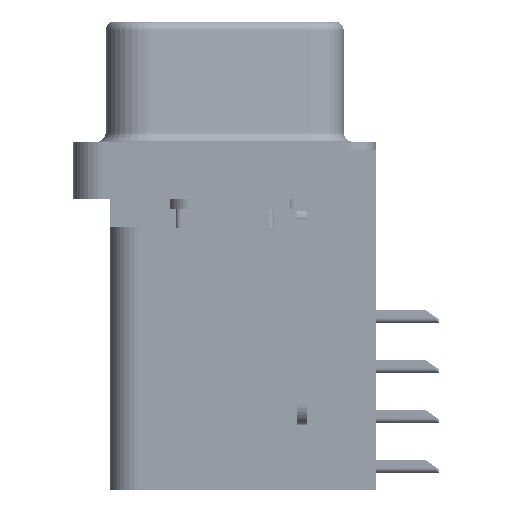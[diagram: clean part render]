
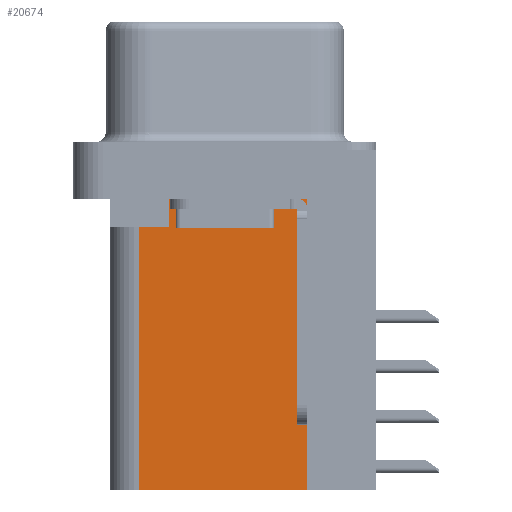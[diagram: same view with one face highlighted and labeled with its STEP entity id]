
A CAD part, left-side view. The second image highlights one B-rep face of the part: STEP entity #20674.
In plain terms, the highlighted planar face has unit normal (-1, 0, 0).
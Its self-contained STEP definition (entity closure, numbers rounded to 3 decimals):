
#11 = VECTOR ( 'NONE', #14169, 1000. ) ;
#483 = EDGE_CURVE ( 'NONE', #10959, #42456, #28727, .T. ) ;
#543 = LINE ( 'NONE', #10920, #11 ) ;
#1434 = DIRECTION ( 'NONE',  ( 0., 0., 1. ) ) ;
#1807 = CARTESIAN_POINT ( 'NONE',  ( 3.75, 2.85, -2.5 ) ) ;
#3070 = ORIENTED_EDGE ( 'NONE', *, *, #483, .F. ) ;
#3157 = CARTESIAN_POINT ( 'NONE',  ( 3.75, -4.2, -17.3 ) ) ;
#3309 = ORIENTED_EDGE ( 'NONE', *, *, #20589, .T. ) ;
#5395 = EDGE_CURVE ( 'NONE', #41770, #30241, #40877, .T. ) ;
#6801 = PLANE ( 'NONE',  #29331 ) ;
#7003 = EDGE_CURVE ( 'NONE', #41770, #10959, #31390, .T. ) ;
#8115 = CARTESIAN_POINT ( 'NONE',  ( 3.75, -4.2, -17.3 ) ) ;
#9763 = CARTESIAN_POINT ( 'NONE',  ( 3.75, -4.2, -2.5 ) ) ;
#10448 = DIRECTION ( 'NONE',  ( 0., 1., 0. ) ) ;
#10920 = CARTESIAN_POINT ( 'NONE',  ( 3.75, 2.85, -3.9 ) ) ;
#10959 = VERTEX_POINT ( 'NONE', #27523 ) ;
#12571 = CARTESIAN_POINT ( 'NONE',  ( 3.75, -4.2, -2.5 ) ) ;
#12845 = CARTESIAN_POINT ( 'NONE',  ( 3.75, 4.35, -17.3 ) ) ;
#13316 = CARTESIAN_POINT ( 'NONE',  ( 3.75, 2.85, -3.9 ) ) ;
#14169 = DIRECTION ( 'NONE',  ( 0., 0., -1. ) ) ;
#15286 = LINE ( 'NONE', #29751, #15405 ) ;
#15405 = VECTOR ( 'NONE', #10448, 1000. ) ;
#16669 = DIRECTION ( 'NONE',  ( 0., 1., 0. ) ) ;
#19621 = FACE_OUTER_BOUND ( 'NONE', #41971, .T. ) ;
#20589 = EDGE_CURVE ( 'NONE', #30241, #28716, #21363, .T. ) ;
#20674 = ADVANCED_FACE ( 'NONE', ( #19621 ), #6801, .F. ) ;
#21363 = LINE ( 'NONE', #9763, #21682 ) ;
#21682 = VECTOR ( 'NONE', #42004, 1000. ) ;
#22432 = ORIENTED_EDGE ( 'NONE', *, *, #24469, .T. ) ;
#22779 = VERTEX_POINT ( 'NONE', #13316 ) ;
#22908 = EDGE_CURVE ( 'NONE', #28716, #22779, #543, .T. ) ;
#23600 = ORIENTED_EDGE ( 'NONE', *, *, #5395, .T. ) ;
#24469 = EDGE_CURVE ( 'NONE', #22779, #42456, #15286, .T. ) ;
#25425 = CARTESIAN_POINT ( 'NONE',  ( 3.75, -4.2, -17.3 ) ) ;
#27523 = CARTESIAN_POINT ( 'NONE',  ( 3.75, 4.35, -17.3 ) ) ;
#28716 = VERTEX_POINT ( 'NONE', #1807 ) ;
#28727 = LINE ( 'NONE', #12845, #28813 ) ;
#28813 = VECTOR ( 'NONE', #31894, 1000. ) ;
#28896 = DIRECTION ( 'NONE',  ( 0., 1., 0. ) ) ;
#29331 = AXIS2_PLACEMENT_3D ( 'NONE', #3157, #36206, #16669 ) ;
#29751 = CARTESIAN_POINT ( 'NONE',  ( 3.75, 0., -3.9 ) ) ;
#30241 = VERTEX_POINT ( 'NONE', #12571 ) ;
#31390 = LINE ( 'NONE', #8115, #31537 ) ;
#31537 = VECTOR ( 'NONE', #28896, 1000. ) ;
#31894 = DIRECTION ( 'NONE',  ( 0., 0., 1. ) ) ;
#32905 = CARTESIAN_POINT ( 'NONE',  ( 3.75, -4.2, -17.3 ) ) ;
#36206 = DIRECTION ( 'NONE',  ( 1., 0., 0. ) ) ;
#37479 = CARTESIAN_POINT ( 'NONE',  ( 3.75, 4.35, -3.9 ) ) ;
#39204 = ORIENTED_EDGE ( 'NONE', *, *, #7003, .F. ) ;
#39321 = ORIENTED_EDGE ( 'NONE', *, *, #22908, .T. ) ;
#40799 = VECTOR ( 'NONE', #1434, 1000. ) ;
#40877 = LINE ( 'NONE', #32905, #40799 ) ;
#41770 = VERTEX_POINT ( 'NONE', #25425 ) ;
#41971 = EDGE_LOOP ( 'NONE', ( #3309, #39321, #22432, #3070, #39204, #23600 ) ) ;
#42004 = DIRECTION ( 'NONE',  ( 0., 1., 0. ) ) ;
#42456 = VERTEX_POINT ( 'NONE', #37479 ) ;
